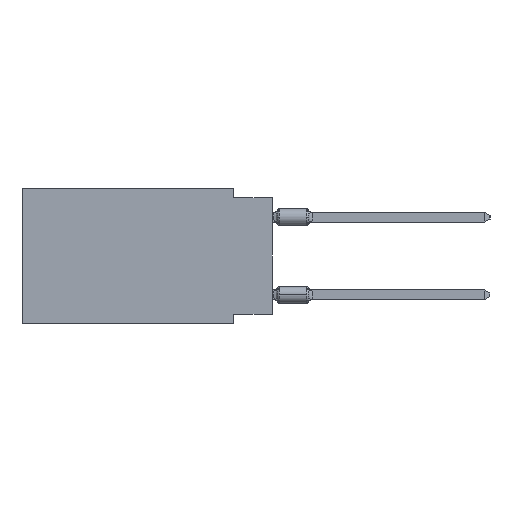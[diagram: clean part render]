
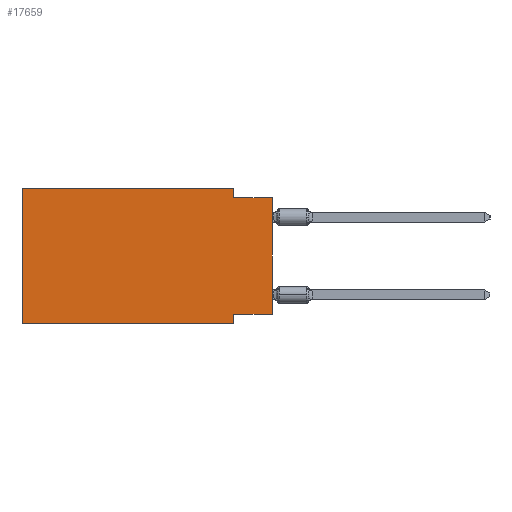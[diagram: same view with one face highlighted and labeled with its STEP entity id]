
A CAD part, left-side view. The second image highlights one B-rep face of the part: STEP entity #17659.
In plain terms, the highlighted planar face has unit normal (-1, 0, 0).
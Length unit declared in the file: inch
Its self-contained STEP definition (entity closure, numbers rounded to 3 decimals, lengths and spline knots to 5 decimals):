
#907 = CARTESIAN_POINT ( 'NONE',  ( 0., 0.645, -0.35 ) ) ;
#1108 = CARTESIAN_POINT ( 'NONE',  ( 0., 0.1, 0. ) ) ;
#1205 = DIRECTION ( 'NONE',  ( 0., -1., 0. ) ) ;
#2443 = EDGE_CURVE ( 'NONE', #34883, #26980, #31123, .T. ) ;
#3675 = ORIENTED_EDGE ( 'NONE', *, *, #51256, .F. ) ;
#4414 = ORIENTED_EDGE ( 'NONE', *, *, #28826, .F. ) ;
#5929 = VERTEX_POINT ( 'NONE', #25506 ) ;
#7828 = VECTOR ( 'NONE', #8895, 39.37008 ) ;
#8516 = VECTOR ( 'NONE', #20991, 39.37008 ) ;
#8671 = VERTEX_POINT ( 'NONE', #19227 ) ;
#8868 = EDGE_CURVE ( 'NONE', #40658, #29966, #55244, .T. ) ;
#8895 = DIRECTION ( 'NONE',  ( 0., -1., 0. ) ) ;
#10625 = VERTEX_POINT ( 'NONE', #42357 ) ;
#11333 = EDGE_LOOP ( 'NONE', ( #40692, #27190, #3675, #56375, #22096, #46422, #16813, #4414 ) ) ;
#15141 = VECTOR ( 'NONE', #38522, 39.37008 ) ;
#15640 = AXIS2_PLACEMENT_3D ( 'NONE', #33471, #27927, #28798 ) ;
#16332 = CARTESIAN_POINT ( 'NONE',  ( 0., 0.645, 0. ) ) ;
#16813 = ORIENTED_EDGE ( 'NONE', *, *, #22357, .F. ) ;
#17659 = ADVANCED_FACE ( 'NONE', ( #55164 ), #37585, .F. ) ;
#17874 = LINE ( 'NONE', #907, #32208 ) ;
#18849 = CARTESIAN_POINT ( 'NONE',  ( 0., 0.645, 0. ) ) ;
#19179 = VECTOR ( 'NONE', #55260, 39.37008 ) ;
#19227 = CARTESIAN_POINT ( 'NONE',  ( 0., 0.1, -0.325 ) ) ;
#20991 = DIRECTION ( 'NONE',  ( 0., 0., 1. ) ) ;
#22096 = ORIENTED_EDGE ( 'NONE', *, *, #31088, .F. ) ;
#22357 = EDGE_CURVE ( 'NONE', #8671, #5929, #43267, .T. ) ;
#23456 = VERTEX_POINT ( 'NONE', #45482 ) ;
#25506 = CARTESIAN_POINT ( 'NONE',  ( 0., 0.1, -0.35 ) ) ;
#26980 = VERTEX_POINT ( 'NONE', #1108 ) ;
#27190 = ORIENTED_EDGE ( 'NONE', *, *, #48340, .F. ) ;
#27927 = DIRECTION ( 'NONE',  ( 1., 0., 0. ) ) ;
#28798 = DIRECTION ( 'NONE',  ( 0., 0., -1. ) ) ;
#28826 = EDGE_CURVE ( 'NONE', #40658, #8671, #56376, .T. ) ;
#29966 = VERTEX_POINT ( 'NONE', #37572 ) ;
#31088 = EDGE_CURVE ( 'NONE', #23456, #34883, #43531, .T. ) ;
#31123 = LINE ( 'NONE', #39893, #7828 ) ;
#32208 = VECTOR ( 'NONE', #1205, 39.37008 ) ;
#32803 = VECTOR ( 'NONE', #42609, 39.37008 ) ;
#33471 = CARTESIAN_POINT ( 'NONE',  ( 0., 0.645, 0. ) ) ;
#34035 = CARTESIAN_POINT ( 'NONE',  ( 0., 0., -0.325 ) ) ;
#34265 = VECTOR ( 'NONE', #47777, 39.37008 ) ;
#34595 = CARTESIAN_POINT ( 'NONE',  ( 0., 0.1, 0. ) ) ;
#34883 = VERTEX_POINT ( 'NONE', #18849 ) ;
#36990 = VECTOR ( 'NONE', #56740, 39.37008 ) ;
#37572 = CARTESIAN_POINT ( 'NONE',  ( 0., 0., -0.025 ) ) ;
#37585 = PLANE ( 'NONE',  #15640 ) ;
#37639 = CARTESIAN_POINT ( 'NONE',  ( 0., 0., -0.325 ) ) ;
#37958 = CARTESIAN_POINT ( 'NONE',  ( 0., 0., -0.025 ) ) ;
#38522 = DIRECTION ( 'NONE',  ( 0., 0., 1. ) ) ;
#39893 = CARTESIAN_POINT ( 'NONE',  ( 0., 0.645, 0. ) ) ;
#40658 = VERTEX_POINT ( 'NONE', #34035 ) ;
#40692 = ORIENTED_EDGE ( 'NONE', *, *, #8868, .T. ) ;
#41769 = LINE ( 'NONE', #37958, #19179 ) ;
#42357 = CARTESIAN_POINT ( 'NONE',  ( 0., 0.1, -0.025 ) ) ;
#42609 = DIRECTION ( 'NONE',  ( 0., 1., 0. ) ) ;
#43267 = LINE ( 'NONE', #48500, #36990 ) ;
#43531 = LINE ( 'NONE', #16332, #8516 ) ;
#43667 = LINE ( 'NONE', #34595, #34265 ) ;
#45482 = CARTESIAN_POINT ( 'NONE',  ( 0., 0.645, -0.35 ) ) ;
#46422 = ORIENTED_EDGE ( 'NONE', *, *, #47808, .T. ) ;
#47777 = DIRECTION ( 'NONE',  ( 0., 0., -1. ) ) ;
#47808 = EDGE_CURVE ( 'NONE', #23456, #5929, #17874, .T. ) ;
#48340 = EDGE_CURVE ( 'NONE', #10625, #29966, #41769, .T. ) ;
#48500 = CARTESIAN_POINT ( 'NONE',  ( 0., 0.1, -0.35 ) ) ;
#51256 = EDGE_CURVE ( 'NONE', #26980, #10625, #43667, .T. ) ;
#55164 = FACE_OUTER_BOUND ( 'NONE', #11333, .T. ) ;
#55244 = LINE ( 'NONE', #56110, #15141 ) ;
#55260 = DIRECTION ( 'NONE',  ( 0., -1., 0. ) ) ;
#56110 = CARTESIAN_POINT ( 'NONE',  ( 0., 0., 0. ) ) ;
#56375 = ORIENTED_EDGE ( 'NONE', *, *, #2443, .F. ) ;
#56376 = LINE ( 'NONE', #37639, #32803 ) ;
#56740 = DIRECTION ( 'NONE',  ( 0., 0., -1. ) ) ;
